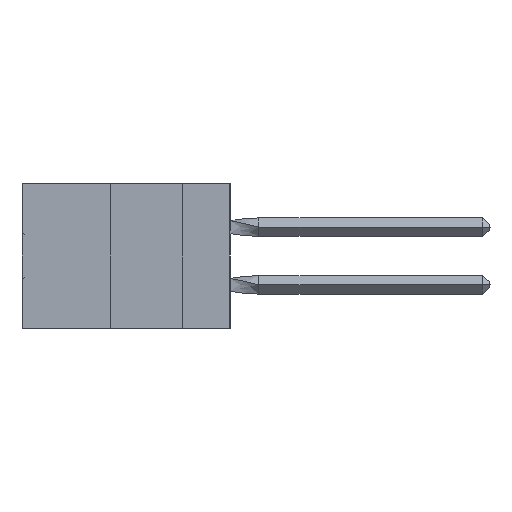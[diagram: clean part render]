
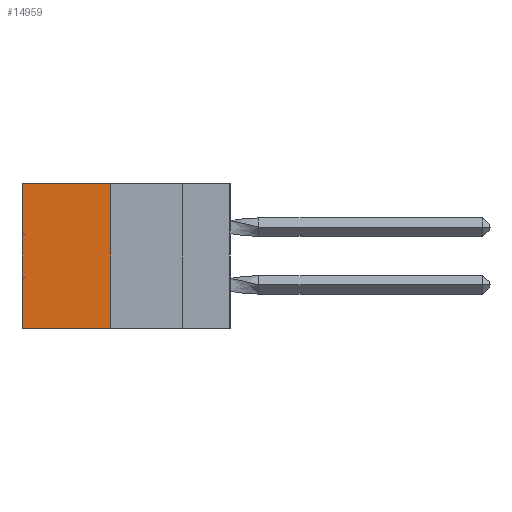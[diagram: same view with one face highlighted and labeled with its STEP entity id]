
A CAD part, left-side view. The second image highlights one B-rep face of the part: STEP entity #14959.
In plain terms, the highlighted planar face has unit normal (-1, 0, 0).
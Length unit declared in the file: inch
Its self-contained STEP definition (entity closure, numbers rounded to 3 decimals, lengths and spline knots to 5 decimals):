
#319 = CARTESIAN_POINT ( 'NONE',  ( 0.305, 0.413, 0. ) ) ;
#600 = VERTEX_POINT ( 'NONE', #319 ) ;
#1581 = DIRECTION ( 'NONE',  ( 1., 0., 0. ) ) ;
#1607 = ORIENTED_EDGE ( 'NONE', *, *, #10725, .F. ) ;
#3123 = CARTESIAN_POINT ( 'NONE',  ( 0.305, 0.413, -0.5 ) ) ;
#3297 = PLANE ( 'NONE',  #41889 ) ;
#3565 = FACE_OUTER_BOUND ( 'NONE', #12479, .T. ) ;
#3950 = DIRECTION ( 'NONE',  ( 0., 1., 0. ) ) ;
#4330 = EDGE_CURVE ( 'NONE', #600, #36713, #36198, .T. ) ;
#4837 = CARTESIAN_POINT ( 'NONE',  ( 0.305, 0.413, 0. ) ) ;
#4880 = VECTOR ( 'NONE', #34226, 39.37008 ) ;
#5599 = ORIENTED_EDGE ( 'NONE', *, *, #16985, .T. ) ;
#6800 = LINE ( 'NONE', #11804, #52464 ) ;
#10725 = EDGE_CURVE ( 'NONE', #600, #11232, #16221, .T. ) ;
#11232 = VERTEX_POINT ( 'NONE', #36908 ) ;
#11804 = CARTESIAN_POINT ( 'NONE',  ( 0.305, 0.413, -0.5 ) ) ;
#11946 = DIRECTION ( 'NONE',  ( 0., 0., -1. ) ) ;
#12479 = EDGE_LOOP ( 'NONE', ( #5599, #32931, #1607, #37233 ) ) ;
#14959 = ADVANCED_FACE ( 'NONE', ( #3565 ), #3297, .F. ) ;
#16221 = LINE ( 'NONE', #36970, #40361 ) ;
#16985 = EDGE_CURVE ( 'NONE', #36713, #44396, #43098, .T. ) ;
#18268 = VECTOR ( 'NONE', #44241, 39.37008 ) ;
#21848 = CARTESIAN_POINT ( 'NONE',  ( 0.305, 0.72, 0. ) ) ;
#32931 = ORIENTED_EDGE ( 'NONE', *, *, #40161, .F. ) ;
#33004 = CARTESIAN_POINT ( 'NONE',  ( 0.305, 0.72, -0.5 ) ) ;
#34080 = CARTESIAN_POINT ( 'NONE',  ( 0.305, 0.72, -0.5 ) ) ;
#34226 = DIRECTION ( 'NONE',  ( 0., 1., 0. ) ) ;
#36198 = LINE ( 'NONE', #4837, #4880 ) ;
#36713 = VERTEX_POINT ( 'NONE', #21848 ) ;
#36908 = CARTESIAN_POINT ( 'NONE',  ( 0.305, 0.413, -0.5 ) ) ;
#36970 = CARTESIAN_POINT ( 'NONE',  ( 0.305, 0.413, -0.5 ) ) ;
#37233 = ORIENTED_EDGE ( 'NONE', *, *, #4330, .T. ) ;
#40161 = EDGE_CURVE ( 'NONE', #11232, #44396, #6800, .T. ) ;
#40361 = VECTOR ( 'NONE', #11946, 39.37008 ) ;
#41889 = AXIS2_PLACEMENT_3D ( 'NONE', #3123, #1581, #52249 ) ;
#43098 = LINE ( 'NONE', #34080, #18268 ) ;
#44241 = DIRECTION ( 'NONE',  ( 0., 0., -1. ) ) ;
#44396 = VERTEX_POINT ( 'NONE', #33004 ) ;
#52249 = DIRECTION ( 'NONE',  ( 0., 0., -1. ) ) ;
#52464 = VECTOR ( 'NONE', #3950, 39.37008 ) ;
